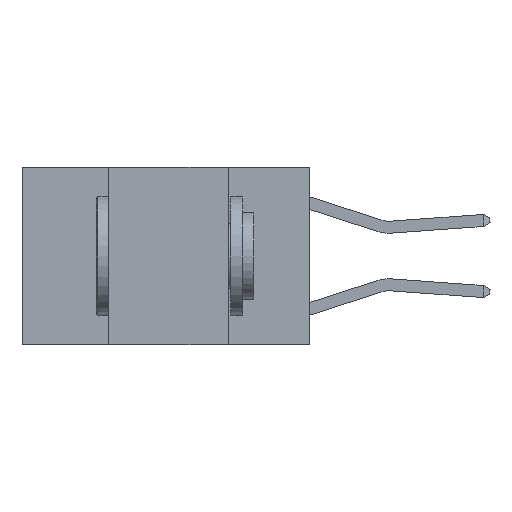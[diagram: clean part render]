
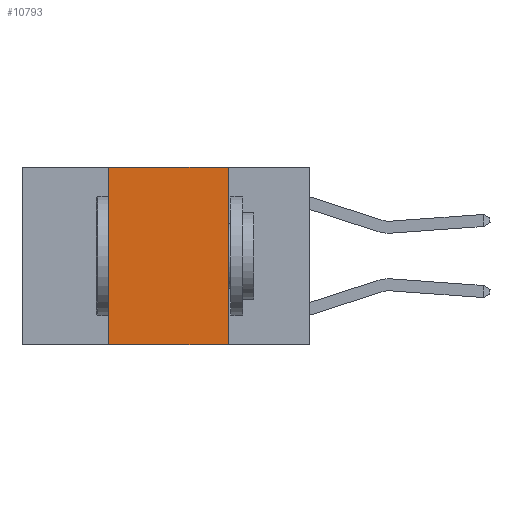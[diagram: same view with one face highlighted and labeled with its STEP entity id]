
A CAD part, left-side view. The second image highlights one B-rep face of the part: STEP entity #10793.
In plain terms, the highlighted planar face has unit normal (-1, 0, 0).
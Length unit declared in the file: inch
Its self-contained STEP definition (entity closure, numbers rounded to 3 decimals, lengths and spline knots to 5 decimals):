
#1085 = CARTESIAN_POINT ( 'NONE',  ( 0., 0.6, 0. ) ) ;
#1750 = VERTEX_POINT ( 'NONE', #4178 ) ;
#2432 = DIRECTION ( 'NONE',  ( 0., 0., -1. ) ) ;
#2881 = CARTESIAN_POINT ( 'NONE',  ( 0., 0.6, 0. ) ) ;
#3282 = EDGE_CURVE ( 'NONE', #10624, #8787, #12795, .T. ) ;
#4178 = CARTESIAN_POINT ( 'NONE',  ( 0., 0.17, 0. ) ) ;
#4586 = EDGE_CURVE ( 'NONE', #10624, #6973, #15319, .T. ) ;
#4722 = VECTOR ( 'NONE', #12773, 39.37008 ) ;
#5052 = CARTESIAN_POINT ( 'NONE',  ( 0., 0.17, -0.37 ) ) ;
#6226 = VECTOR ( 'NONE', #7733, 39.37008 ) ;
#6973 = VERTEX_POINT ( 'NONE', #9917 ) ;
#7403 = DIRECTION ( 'NONE',  ( 0., -1., 0. ) ) ;
#7733 = DIRECTION ( 'NONE',  ( 0., -1., 0. ) ) ;
#8787 = VERTEX_POINT ( 'NONE', #5052 ) ;
#9544 = FACE_OUTER_BOUND ( 'NONE', #14037, .T. ) ;
#9917 = CARTESIAN_POINT ( 'NONE',  ( 0., 0.42, 0. ) ) ;
#10038 = CARTESIAN_POINT ( 'NONE',  ( 0., 0.42, 0. ) ) ;
#10624 = VERTEX_POINT ( 'NONE', #14562 ) ;
#10713 = ORIENTED_EDGE ( 'NONE', *, *, #13176, .F. ) ;
#10793 = ADVANCED_FACE ( 'NONE', ( #9544 ), #14916, .F. ) ;
#11412 = EDGE_CURVE ( 'NONE', #6973, #1750, #15575, .T. ) ;
#11518 = ORIENTED_EDGE ( 'NONE', *, *, #4586, .F. ) ;
#11837 = LINE ( 'NONE', #14462, #14824 ) ;
#12707 = CARTESIAN_POINT ( 'NONE',  ( 0., 0.6, -0.37 ) ) ;
#12773 = DIRECTION ( 'NONE',  ( 0., 0., 1. ) ) ;
#12795 = LINE ( 'NONE', #12707, #13794 ) ;
#12998 = ORIENTED_EDGE ( 'NONE', *, *, #3282, .T. ) ;
#13176 = EDGE_CURVE ( 'NONE', #1750, #8787, #11837, .T. ) ;
#13608 = DIRECTION ( 'NONE',  ( 1., 0., 0. ) ) ;
#13643 = AXIS2_PLACEMENT_3D ( 'NONE', #2881, #13608, #13940 ) ;
#13794 = VECTOR ( 'NONE', #7403, 39.37008 ) ;
#13940 = DIRECTION ( 'NONE',  ( 0., 0., -1. ) ) ;
#14037 = EDGE_LOOP ( 'NONE', ( #10713, #16242, #11518, #12998 ) ) ;
#14462 = CARTESIAN_POINT ( 'NONE',  ( 0., 0.17, 0. ) ) ;
#14562 = CARTESIAN_POINT ( 'NONE',  ( 0., 0.42, -0.37 ) ) ;
#14824 = VECTOR ( 'NONE', #2432, 39.37008 ) ;
#14916 = PLANE ( 'NONE',  #13643 ) ;
#15319 = LINE ( 'NONE', #10038, #4722 ) ;
#15575 = LINE ( 'NONE', #1085, #6226 ) ;
#16242 = ORIENTED_EDGE ( 'NONE', *, *, #11412, .F. ) ;
